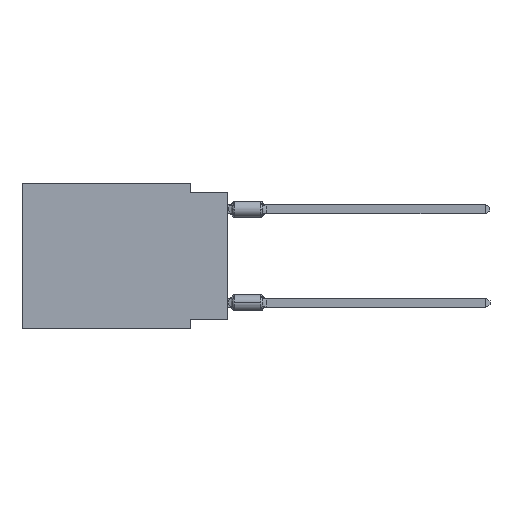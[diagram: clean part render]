
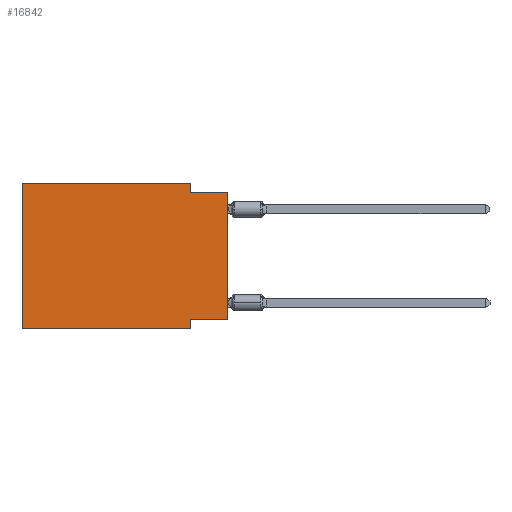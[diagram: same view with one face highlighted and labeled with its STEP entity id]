
A CAD part, left-side view. The second image highlights one B-rep face of the part: STEP entity #16842.
In plain terms, the highlighted planar face has unit normal (-1, 0, 0).
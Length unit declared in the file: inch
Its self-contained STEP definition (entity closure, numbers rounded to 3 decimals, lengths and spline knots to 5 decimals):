
#15 = LINE ( 'NONE', #207, #159 ) ;
#61 = CARTESIAN_POINT ( 'NONE',  ( 0., 0.1, -0.365 ) ) ;
#159 = VECTOR ( 'NONE', #15990, 39.37008 ) ;
#207 = CARTESIAN_POINT ( 'NONE',  ( 0., 0., -0.365 ) ) ;
#660 = DIRECTION ( 'NONE',  ( 0., 0., -1. ) ) ;
#899 = LINE ( 'NONE', #10777, #13856 ) ;
#1533 = CARTESIAN_POINT ( 'NONE',  ( 0., 0.55, 0. ) ) ;
#1697 = CARTESIAN_POINT ( 'NONE',  ( 0., 0.1, 0. ) ) ;
#1897 = DIRECTION ( 'NONE',  ( 1., 0., 0. ) ) ;
#1939 = LINE ( 'NONE', #17629, #17450 ) ;
#2165 = CARTESIAN_POINT ( 'NONE',  ( 0., 0., -0.365 ) ) ;
#2291 = VERTEX_POINT ( 'NONE', #61 ) ;
#2526 = ORIENTED_EDGE ( 'NONE', *, *, #4698, .F. ) ;
#2535 = DIRECTION ( 'NONE',  ( 0., -1., 0. ) ) ;
#2583 = ORIENTED_EDGE ( 'NONE', *, *, #9583, .F. ) ;
#3154 = VERTEX_POINT ( 'NONE', #15890 ) ;
#3166 = DIRECTION ( 'NONE',  ( 0., -1., 0. ) ) ;
#3167 = ORIENTED_EDGE ( 'NONE', *, *, #10547, .F. ) ;
#4082 = CARTESIAN_POINT ( 'NONE',  ( 0., 0.55, 0. ) ) ;
#4160 = LINE ( 'NONE', #1533, #16350 ) ;
#4698 = EDGE_CURVE ( 'NONE', #2291, #5059, #17279, .T. ) ;
#5059 = VERTEX_POINT ( 'NONE', #11249 ) ;
#5311 = CARTESIAN_POINT ( 'NONE',  ( 0., 0.55, -0.39 ) ) ;
#5343 = EDGE_CURVE ( 'NONE', #10026, #5903, #899, .T. ) ;
#5564 = DIRECTION ( 'NONE',  ( 0., 0., 1. ) ) ;
#5903 = VERTEX_POINT ( 'NONE', #1697 ) ;
#5911 = EDGE_CURVE ( 'NONE', #5903, #10553, #12029, .T. ) ;
#6101 = PLANE ( 'NONE',  #9936 ) ;
#6147 = EDGE_CURVE ( 'NONE', #15238, #3154, #10618, .T. ) ;
#6522 = VECTOR ( 'NONE', #17829, 39.37008 ) ;
#7051 = CARTESIAN_POINT ( 'NONE',  ( 0., 0.1, -0.025 ) ) ;
#8502 = EDGE_LOOP ( 'NONE', ( #8678, #13850, #18190, #8592, #2583, #12019, #2526, #3167 ) ) ;
#8592 = ORIENTED_EDGE ( 'NONE', *, *, #5343, .F. ) ;
#8678 = ORIENTED_EDGE ( 'NONE', *, *, #6147, .T. ) ;
#8859 = FACE_OUTER_BOUND ( 'NONE', #8502, .T. ) ;
#9583 = EDGE_CURVE ( 'NONE', #16174, #10026, #4160, .T. ) ;
#9688 = LINE ( 'NONE', #15409, #14270 ) ;
#9936 = AXIS2_PLACEMENT_3D ( 'NONE', #11858, #1897, #11766 ) ;
#10026 = VERTEX_POINT ( 'NONE', #4082 ) ;
#10547 = EDGE_CURVE ( 'NONE', #15238, #2291, #15, .T. ) ;
#10553 = VERTEX_POINT ( 'NONE', #7051 ) ;
#10618 = LINE ( 'NONE', #15019, #6522 ) ;
#10777 = CARTESIAN_POINT ( 'NONE',  ( 0., 0.55, 0. ) ) ;
#10941 = EDGE_CURVE ( 'NONE', #16174, #5059, #9688, .T. ) ;
#11249 = CARTESIAN_POINT ( 'NONE',  ( 0., 0.1, -0.39 ) ) ;
#11312 = VECTOR ( 'NONE', #15591, 39.37008 ) ;
#11766 = DIRECTION ( 'NONE',  ( 0., 0., -1. ) ) ;
#11858 = CARTESIAN_POINT ( 'NONE',  ( 0., 0.55, 0. ) ) ;
#12019 = ORIENTED_EDGE ( 'NONE', *, *, #10941, .T. ) ;
#12029 = LINE ( 'NONE', #13538, #14957 ) ;
#13538 = CARTESIAN_POINT ( 'NONE',  ( 0., 0.1, 0. ) ) ;
#13850 = ORIENTED_EDGE ( 'NONE', *, *, #17908, .F. ) ;
#13856 = VECTOR ( 'NONE', #15094, 39.37008 ) ;
#14270 = VECTOR ( 'NONE', #2535, 39.37008 ) ;
#14957 = VECTOR ( 'NONE', #660, 39.37008 ) ;
#15019 = CARTESIAN_POINT ( 'NONE',  ( 0., 0., 0. ) ) ;
#15094 = DIRECTION ( 'NONE',  ( 0., -1., 0. ) ) ;
#15238 = VERTEX_POINT ( 'NONE', #2165 ) ;
#15409 = CARTESIAN_POINT ( 'NONE',  ( 0., 0.55, -0.39 ) ) ;
#15591 = DIRECTION ( 'NONE',  ( 0., 0., -1. ) ) ;
#15890 = CARTESIAN_POINT ( 'NONE',  ( 0., 0., -0.025 ) ) ;
#15990 = DIRECTION ( 'NONE',  ( 0., 1., 0. ) ) ;
#16174 = VERTEX_POINT ( 'NONE', #5311 ) ;
#16350 = VECTOR ( 'NONE', #5564, 39.37008 ) ;
#16842 = ADVANCED_FACE ( 'NONE', ( #8859 ), #6101, .F. ) ;
#17187 = CARTESIAN_POINT ( 'NONE',  ( 0., 0.1, -0.39 ) ) ;
#17279 = LINE ( 'NONE', #17187, #11312 ) ;
#17450 = VECTOR ( 'NONE', #3166, 39.37008 ) ;
#17629 = CARTESIAN_POINT ( 'NONE',  ( 0., 0., -0.025 ) ) ;
#17829 = DIRECTION ( 'NONE',  ( 0., 0., 1. ) ) ;
#17908 = EDGE_CURVE ( 'NONE', #10553, #3154, #1939, .T. ) ;
#18190 = ORIENTED_EDGE ( 'NONE', *, *, #5911, .F. ) ;
